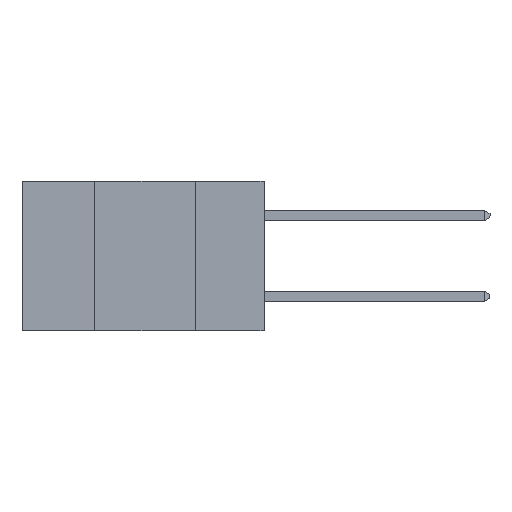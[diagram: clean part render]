
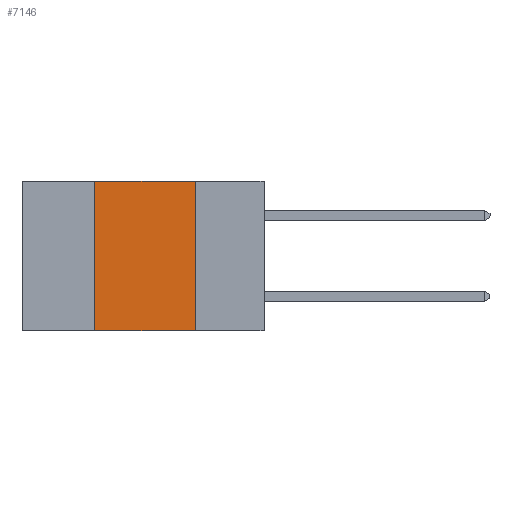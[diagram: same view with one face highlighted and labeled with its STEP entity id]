
A CAD part, left-side view. The second image highlights one B-rep face of the part: STEP entity #7146.
In plain terms, the highlighted planar face has unit normal (-1, 0, 0).
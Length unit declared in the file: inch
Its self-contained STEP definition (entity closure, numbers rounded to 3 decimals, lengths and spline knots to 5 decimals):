
#752 = VERTEX_POINT ( 'NONE', #7013 ) ;
#865 = CARTESIAN_POINT ( 'NONE',  ( 0., 0.6, 0. ) ) ;
#1143 = VECTOR ( 'NONE', #10851, 39.37008 ) ;
#1367 = ORIENTED_EDGE ( 'NONE', *, *, #13395, .F. ) ;
#2094 = DIRECTION ( 'NONE',  ( 1., 0., 0. ) ) ;
#2596 = CARTESIAN_POINT ( 'NONE',  ( 0., 0.6, 0. ) ) ;
#2648 = CARTESIAN_POINT ( 'NONE',  ( 0., 0.17, 0. ) ) ;
#2798 = EDGE_LOOP ( 'NONE', ( #1367, #11833, #7821, #6853 ) ) ;
#3754 = VERTEX_POINT ( 'NONE', #9470 ) ;
#3860 = LINE ( 'NONE', #6696, #9709 ) ;
#5015 = CARTESIAN_POINT ( 'NONE',  ( 0., 0.42, 0. ) ) ;
#5669 = PLANE ( 'NONE',  #11348 ) ;
#5750 = EDGE_CURVE ( 'NONE', #7025, #3754, #3860, .T. ) ;
#5867 = DIRECTION ( 'NONE',  ( 0., 0., 1. ) ) ;
#6076 = EDGE_CURVE ( 'NONE', #10076, #752, #11484, .T. ) ;
#6653 = LINE ( 'NONE', #11688, #15245 ) ;
#6696 = CARTESIAN_POINT ( 'NONE',  ( 0., 0.6, -0.37 ) ) ;
#6853 = ORIENTED_EDGE ( 'NONE', *, *, #5750, .T. ) ;
#7013 = CARTESIAN_POINT ( 'NONE',  ( 0., 0.17, 0. ) ) ;
#7025 = VERTEX_POINT ( 'NONE', #8975 ) ;
#7146 = ADVANCED_FACE ( 'NONE', ( #7777 ), #5669, .F. ) ;
#7777 = FACE_OUTER_BOUND ( 'NONE', #2798, .T. ) ;
#7821 = ORIENTED_EDGE ( 'NONE', *, *, #13873, .F. ) ;
#7983 = DIRECTION ( 'NONE',  ( 0., 0., -1. ) ) ;
#8440 = DIRECTION ( 'NONE',  ( 0., -1., 0. ) ) ;
#8975 = CARTESIAN_POINT ( 'NONE',  ( 0., 0.42, -0.37 ) ) ;
#9470 = CARTESIAN_POINT ( 'NONE',  ( 0., 0.17, -0.37 ) ) ;
#9709 = VECTOR ( 'NONE', #13732, 39.37008 ) ;
#10076 = VERTEX_POINT ( 'NONE', #5015 ) ;
#10201 = LINE ( 'NONE', #2648, #1143 ) ;
#10851 = DIRECTION ( 'NONE',  ( 0., 0., -1. ) ) ;
#11136 = VECTOR ( 'NONE', #8440, 39.37008 ) ;
#11348 = AXIS2_PLACEMENT_3D ( 'NONE', #865, #2094, #7983 ) ;
#11484 = LINE ( 'NONE', #2596, #11136 ) ;
#11688 = CARTESIAN_POINT ( 'NONE',  ( 0., 0.42, 0. ) ) ;
#11833 = ORIENTED_EDGE ( 'NONE', *, *, #6076, .F. ) ;
#13395 = EDGE_CURVE ( 'NONE', #752, #3754, #10201, .T. ) ;
#13732 = DIRECTION ( 'NONE',  ( 0., -1., 0. ) ) ;
#13873 = EDGE_CURVE ( 'NONE', #7025, #10076, #6653, .T. ) ;
#15245 = VECTOR ( 'NONE', #5867, 39.37008 ) ;
